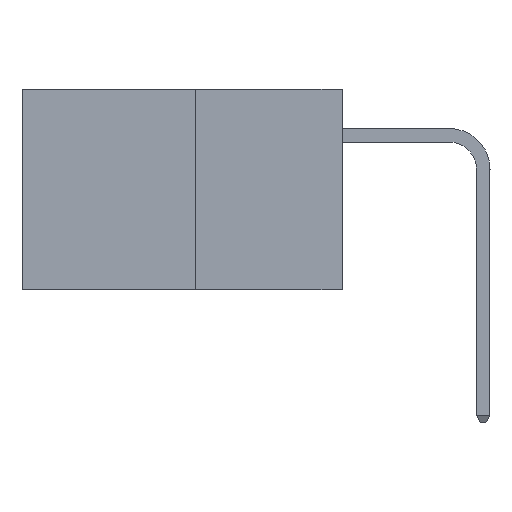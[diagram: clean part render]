
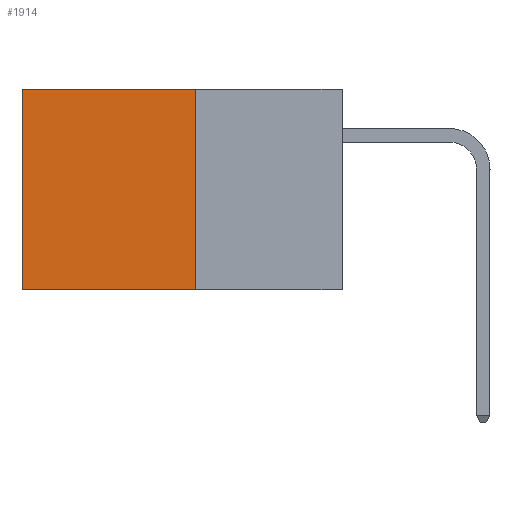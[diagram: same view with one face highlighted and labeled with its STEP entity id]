
A CAD part, left-side view. The second image highlights one B-rep face of the part: STEP entity #1914.
In plain terms, the highlighted planar face has unit normal (-1, 0, 0).
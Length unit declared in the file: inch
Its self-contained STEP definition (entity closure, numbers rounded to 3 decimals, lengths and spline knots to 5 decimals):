
#123 = VERTEX_POINT ( 'NONE', #6194 ) ;
#300 = VERTEX_POINT ( 'NONE', #8023 ) ;
#493 = CARTESIAN_POINT ( 'NONE',  ( 0.277, 0.27, -0.37 ) ) ;
#643 = LINE ( 'NONE', #493, #9266 ) ;
#823 = CARTESIAN_POINT ( 'NONE',  ( 0.277, 0.59, 0. ) ) ;
#1131 = EDGE_CURVE ( 'NONE', #9448, #123, #643, .T. ) ;
#1146 = ORIENTED_EDGE ( 'NONE', *, *, #1721, .T. ) ;
#1513 = DIRECTION ( 'NONE',  ( 0., 0., -1. ) ) ;
#1721 = EDGE_CURVE ( 'NONE', #300, #7833, #9210, .T. ) ;
#1725 = CARTESIAN_POINT ( 'NONE',  ( 0.277, 0.59, -0.37 ) ) ;
#1914 = ADVANCED_FACE ( 'NONE', ( #2730 ), #6061, .F. ) ;
#2728 = EDGE_LOOP ( 'NONE', ( #4738, #6615, #4733, #1146 ) ) ;
#2730 = FACE_OUTER_BOUND ( 'NONE', #2728, .T. ) ;
#3990 = EDGE_CURVE ( 'NONE', #300, #9448, #4844, .T. ) ;
#4733 = ORIENTED_EDGE ( 'NONE', *, *, #3990, .F. ) ;
#4738 = ORIENTED_EDGE ( 'NONE', *, *, #6273, .T. ) ;
#4844 = LINE ( 'NONE', #6517, #8770 ) ;
#5089 = DIRECTION ( 'NONE',  ( 0., 0., -1. ) ) ;
#5142 = DIRECTION ( 'NONE',  ( 1., 0., 0. ) ) ;
#5237 = AXIS2_PLACEMENT_3D ( 'NONE', #6495, #5142, #5089 ) ;
#5321 = VECTOR ( 'NONE', #9481, 39.37008 ) ;
#5999 = VECTOR ( 'NONE', #1513, 39.37008 ) ;
#6061 = PLANE ( 'NONE',  #5237 ) ;
#6194 = CARTESIAN_POINT ( 'NONE',  ( 0.277, 0.59, -0.37 ) ) ;
#6273 = EDGE_CURVE ( 'NONE', #7833, #123, #8093, .T. ) ;
#6495 = CARTESIAN_POINT ( 'NONE',  ( 0.277, 0.27, -0.37 ) ) ;
#6517 = CARTESIAN_POINT ( 'NONE',  ( 0.277, 0.27, -0.37 ) ) ;
#6539 = DIRECTION ( 'NONE',  ( 0., 0., -1. ) ) ;
#6615 = ORIENTED_EDGE ( 'NONE', *, *, #1131, .F. ) ;
#7374 = DIRECTION ( 'NONE',  ( 0., 1., 0. ) ) ;
#7833 = VERTEX_POINT ( 'NONE', #823 ) ;
#8023 = CARTESIAN_POINT ( 'NONE',  ( 0.277, 0.27, 0. ) ) ;
#8093 = LINE ( 'NONE', #1725, #5999 ) ;
#8770 = VECTOR ( 'NONE', #6539, 39.37008 ) ;
#8799 = CARTESIAN_POINT ( 'NONE',  ( 0.277, 0.27, -0.37 ) ) ;
#9210 = LINE ( 'NONE', #9540, #5321 ) ;
#9266 = VECTOR ( 'NONE', #7374, 39.37008 ) ;
#9448 = VERTEX_POINT ( 'NONE', #8799 ) ;
#9481 = DIRECTION ( 'NONE',  ( 0., 1., 0. ) ) ;
#9540 = CARTESIAN_POINT ( 'NONE',  ( 0.277, 0.27, 0. ) ) ;
